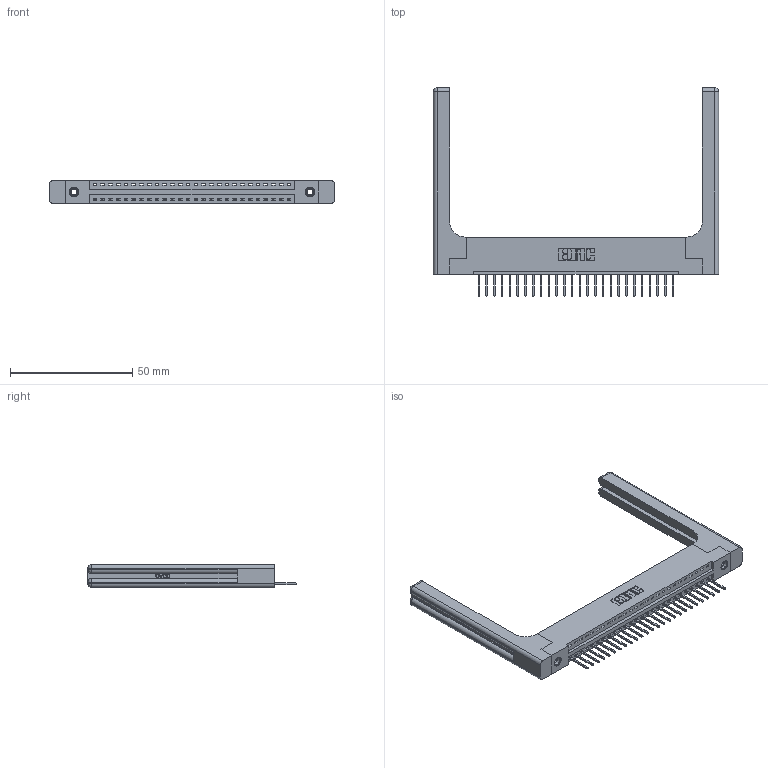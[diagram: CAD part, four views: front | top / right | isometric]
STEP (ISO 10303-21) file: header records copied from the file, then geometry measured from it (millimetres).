
FILE_DESCRIPTION (( 'STEP AP203' ), '1' );
FILE_NAME ('346-026-526-158.STEP', '2022-05-06T02:43:58', ( '' ), ( '' ), 'SwSTEP 2.0', 'SolidWorks 2020', '' );
FILE_SCHEMA (( 'CONFIG_CONTROL_DESIGN' ));
Length unit declared in the file: inch
Products named in the file (5): 345-292-001_345-293-126; 345-250-001_345-250-001-102; 346-220-058_345-220-058; 346 Part_Flush Mounting Lugs - 0.156 Dia-TH; 346-026-526-158
Assembly tree (31 placements, depth 2):
  346-026-526-158
    346 Part_Flush Mounting Lugs - 0.156 Dia-TH
    345-292-001_345-293-126  x26
    345-250-001_345-250-001-102  x2
    346-220-058_345-220-058  x2
Bounding box: 116.61 x 85.09 x 9.4 mm (x, y, z)
Volume: 18531.6 mm3; surface area: 18769 mm2
Topology: 31 solids, 31 shells, 1900 faces, 5607 edges, 3682 vertices
Faces by surface type: plane 1278, cylinder 562, bspline 36, cone 12, sphere 8, torus 4
Entity records: 23906 total; most frequent: CARTESIAN_POINT 5085, ORIENTED_EDGE 3840, DIRECTION 3436, EDGE_CURVE 1920, LINE 1592, VECTOR 1592, VERTEX_POINT 1270, AXIS2_PLACEMENT_3D 922
